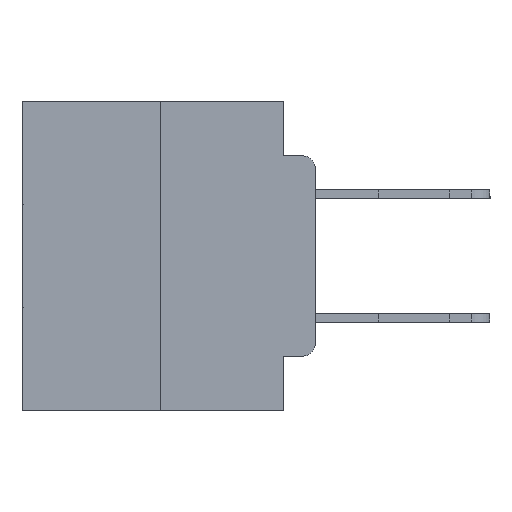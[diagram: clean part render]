
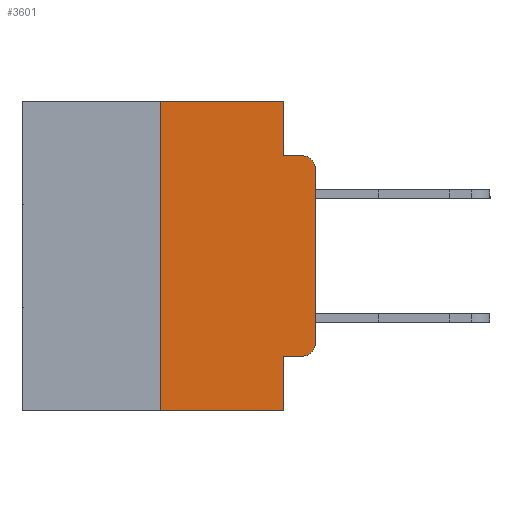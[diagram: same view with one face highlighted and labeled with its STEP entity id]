
A CAD part, left-side view. The second image highlights one B-rep face of the part: STEP entity #3601.
In plain terms, the highlighted planar face has unit normal (-1, 0, 0).
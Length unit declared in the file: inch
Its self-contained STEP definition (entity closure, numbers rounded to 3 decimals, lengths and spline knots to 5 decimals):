
#244 = DIRECTION ( 'NONE',  ( 0., -1., 0. ) ) ;
#608 = ORIENTED_EDGE ( 'NONE', *, *, #15287, .F. ) ;
#1098 = EDGE_CURVE ( 'NONE', #6549, #10734, #17011, .T. ) ;
#2255 = DIRECTION ( 'NONE',  ( 0., -1., 0. ) ) ;
#2290 = CARTESIAN_POINT ( 'NONE',  ( 0., 0.02, -0.3915 ) ) ;
#2746 = DIRECTION ( 'NONE',  ( -1., 0., 0. ) ) ;
#3359 = ORIENTED_EDGE ( 'NONE', *, *, #1098, .F. ) ;
#3523 = CARTESIAN_POINT ( 'NONE',  ( 0., 0.051, 0. ) ) ;
#3537 = AXIS2_PLACEMENT_3D ( 'NONE', #2290, #10981, #10946 ) ;
#3601 = ADVANCED_FACE ( 'NONE', ( #17595 ), #5964, .F. ) ;
#3703 = CARTESIAN_POINT ( 'NONE',  ( 0., 0.051, -0.4115 ) ) ;
#3813 = VECTOR ( 'NONE', #244, 39.37008 ) ;
#4719 = ORIENTED_EDGE ( 'NONE', *, *, #21362, .T. ) ;
#5698 = DIRECTION ( 'NONE',  ( 1., 0., 0. ) ) ;
#5790 = CARTESIAN_POINT ( 'NONE',  ( 0., 0.473, 0. ) ) ;
#5872 = DIRECTION ( 'NONE',  ( 0., 0., -1. ) ) ;
#5874 = DIRECTION ( 'NONE',  ( 0., 0., -1. ) ) ;
#5964 = PLANE ( 'NONE',  #10301 ) ;
#5976 = CARTESIAN_POINT ( 'NONE',  ( 0., 0.051, 0. ) ) ;
#6549 = VERTEX_POINT ( 'NONE', #17891 ) ;
#6586 = CIRCLE ( 'NONE', #3537, 0.02 ) ;
#6685 = EDGE_CURVE ( 'NONE', #16921, #22267, #6586, .T. ) ;
#6920 = VERTEX_POINT ( 'NONE', #24998 ) ;
#7314 = VERTEX_POINT ( 'NONE', #19185 ) ;
#7472 = ORIENTED_EDGE ( 'NONE', *, *, #8126, .T. ) ;
#7652 = DIRECTION ( 'NONE',  ( 0., 0., 1. ) ) ;
#7685 = CARTESIAN_POINT ( 'NONE',  ( 0., 0.25, -0.5 ) ) ;
#8126 = EDGE_CURVE ( 'NONE', #21825, #16921, #20867, .T. ) ;
#9319 = VECTOR ( 'NONE', #5874, 39.37008 ) ;
#9541 = EDGE_CURVE ( 'NONE', #21825, #21425, #18744, .T. ) ;
#9726 = ORIENTED_EDGE ( 'NONE', *, *, #10972, .F. ) ;
#10301 = AXIS2_PLACEMENT_3D ( 'NONE', #5790, #5698, #5872 ) ;
#10337 = VECTOR ( 'NONE', #7652, 39.37008 ) ;
#10717 = AXIS2_PLACEMENT_3D ( 'NONE', #15578, #2746, #17699 ) ;
#10734 = VERTEX_POINT ( 'NONE', #14930 ) ;
#10744 = CARTESIAN_POINT ( 'NONE',  ( 0., 0.473, -0.5 ) ) ;
#10946 = DIRECTION ( 'NONE',  ( 0., 0., -1. ) ) ;
#10972 = EDGE_CURVE ( 'NONE', #23779, #6549, #16015, .T. ) ;
#10981 = DIRECTION ( 'NONE',  ( -1., 0., 0. ) ) ;
#10986 = CARTESIAN_POINT ( 'NONE',  ( 0., 0.051, -0.4115 ) ) ;
#12056 = VECTOR ( 'NONE', #21405, 39.37008 ) ;
#12101 = CIRCLE ( 'NONE', #10717, 0.02 ) ;
#12411 = EDGE_CURVE ( 'NONE', #10734, #7314, #26996, .T. ) ;
#12721 = ORIENTED_EDGE ( 'NONE', *, *, #12411, .F. ) ;
#12742 = VECTOR ( 'NONE', #12892, 39.37008 ) ;
#12892 = DIRECTION ( 'NONE',  ( 0., -1., 0. ) ) ;
#13789 = VECTOR ( 'NONE', #18444, 39.37008 ) ;
#14930 = CARTESIAN_POINT ( 'NONE',  ( 0., 0.051, 0. ) ) ;
#15287 = EDGE_CURVE ( 'NONE', #7314, #23785, #21866, .T. ) ;
#15578 = CARTESIAN_POINT ( 'NONE',  ( 0., 0.02, -0.1085 ) ) ;
#15730 = ORIENTED_EDGE ( 'NONE', *, *, #18103, .T. ) ;
#16015 = LINE ( 'NONE', #22479, #10337 ) ;
#16241 = CARTESIAN_POINT ( 'NONE',  ( 0., 0.02, -0.0885 ) ) ;
#16321 = DIRECTION ( 'NONE',  ( 0., 0., 1. ) ) ;
#16668 = EDGE_CURVE ( 'NONE', #6920, #23785, #12101, .T. ) ;
#16921 = VERTEX_POINT ( 'NONE', #22746 ) ;
#17011 = LINE ( 'NONE', #27697, #12056 ) ;
#17209 = CARTESIAN_POINT ( 'NONE',  ( 0., 0.051, -0.0885 ) ) ;
#17595 = FACE_OUTER_BOUND ( 'NONE', #23618, .T. ) ;
#17699 = DIRECTION ( 'NONE',  ( 0., 0., -1. ) ) ;
#17891 = CARTESIAN_POINT ( 'NONE',  ( 0., 0.25, 0. ) ) ;
#18103 = EDGE_CURVE ( 'NONE', #22267, #6920, #26554, .T. ) ;
#18366 = CARTESIAN_POINT ( 'NONE',  ( 0., 0., 0. ) ) ;
#18444 = DIRECTION ( 'NONE',  ( 0., 0., -1. ) ) ;
#18744 = LINE ( 'NONE', #3523, #13789 ) ;
#19185 = CARTESIAN_POINT ( 'NONE',  ( 0., 0.051, -0.0885 ) ) ;
#19388 = CARTESIAN_POINT ( 'NONE',  ( 0., 0.051, -0.5 ) ) ;
#20607 = VECTOR ( 'NONE', #16321, 39.37008 ) ;
#20867 = LINE ( 'NONE', #10986, #3813 ) ;
#21362 = EDGE_CURVE ( 'NONE', #23779, #21425, #24088, .T. ) ;
#21405 = DIRECTION ( 'NONE',  ( 0., -1., 0. ) ) ;
#21425 = VERTEX_POINT ( 'NONE', #19388 ) ;
#21825 = VERTEX_POINT ( 'NONE', #3703 ) ;
#21866 = LINE ( 'NONE', #17209, #26180 ) ;
#22267 = VERTEX_POINT ( 'NONE', #26456 ) ;
#22479 = CARTESIAN_POINT ( 'NONE',  ( 0., 0.25, 0. ) ) ;
#22746 = CARTESIAN_POINT ( 'NONE',  ( 0., 0.02, -0.4115 ) ) ;
#23618 = EDGE_LOOP ( 'NONE', ( #15730, #27043, #608, #12721, #3359, #9726, #4719, #24098, #7472, #27733 ) ) ;
#23779 = VERTEX_POINT ( 'NONE', #7685 ) ;
#23785 = VERTEX_POINT ( 'NONE', #16241 ) ;
#24088 = LINE ( 'NONE', #10744, #12742 ) ;
#24098 = ORIENTED_EDGE ( 'NONE', *, *, #9541, .F. ) ;
#24998 = CARTESIAN_POINT ( 'NONE',  ( 0., 0., -0.1085 ) ) ;
#26180 = VECTOR ( 'NONE', #2255, 39.37008 ) ;
#26456 = CARTESIAN_POINT ( 'NONE',  ( 0., 0., -0.3915 ) ) ;
#26554 = LINE ( 'NONE', #18366, #20607 ) ;
#26996 = LINE ( 'NONE', #5976, #9319 ) ;
#27043 = ORIENTED_EDGE ( 'NONE', *, *, #16668, .T. ) ;
#27697 = CARTESIAN_POINT ( 'NONE',  ( 0., 0.473, 0. ) ) ;
#27733 = ORIENTED_EDGE ( 'NONE', *, *, #6685, .T. ) ;
